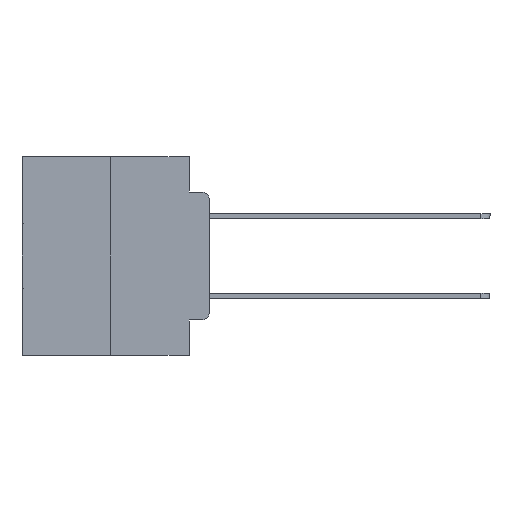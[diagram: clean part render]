
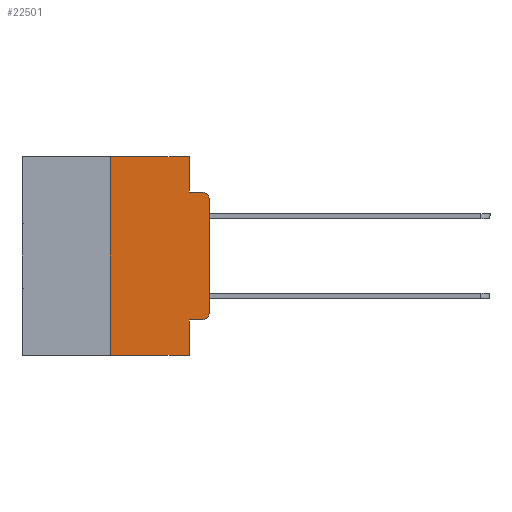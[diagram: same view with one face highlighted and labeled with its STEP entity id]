
A CAD part, left-side view. The second image highlights one B-rep face of the part: STEP entity #22501.
In plain terms, the highlighted planar face has unit normal (-1, 0, 0).
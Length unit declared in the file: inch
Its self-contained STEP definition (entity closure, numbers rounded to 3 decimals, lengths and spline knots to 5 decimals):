
#284 = CARTESIAN_POINT ( 'NONE',  ( 0., 0.051, -0.4115 ) ) ;
#371 = ORIENTED_EDGE ( 'NONE', *, *, #9940, .F. ) ;
#402 = VERTEX_POINT ( 'NONE', #22091 ) ;
#1548 = DIRECTION ( 'NONE',  ( 1., 0., 0. ) ) ;
#1615 = CIRCLE ( 'NONE', #17245, 0.02 ) ;
#2253 = EDGE_CURVE ( 'NONE', #23236, #7248, #24080, .T. ) ;
#2293 = ORIENTED_EDGE ( 'NONE', *, *, #23768, .T. ) ;
#2400 = EDGE_CURVE ( 'NONE', #23425, #27001, #1615, .T. ) ;
#2680 = ORIENTED_EDGE ( 'NONE', *, *, #15857, .F. ) ;
#2745 = DIRECTION ( 'NONE',  ( 0., -1., 0. ) ) ;
#4505 = LINE ( 'NONE', #23793, #22493 ) ;
#5071 = DIRECTION ( 'NONE',  ( 0., -1., 0. ) ) ;
#5350 = VECTOR ( 'NONE', #19750, 39.37008 ) ;
#6028 = ORIENTED_EDGE ( 'NONE', *, *, #2253, .F. ) ;
#7029 = CARTESIAN_POINT ( 'NONE',  ( 0., 0.051, 0. ) ) ;
#7248 = VERTEX_POINT ( 'NONE', #28338 ) ;
#7427 = DIRECTION ( 'NONE',  ( 0., 0., 1. ) ) ;
#7777 = VERTEX_POINT ( 'NONE', #9483 ) ;
#8182 = LINE ( 'NONE', #23609, #13715 ) ;
#9483 = CARTESIAN_POINT ( 'NONE',  ( 0., 0.051, -0.4115 ) ) ;
#9668 = DIRECTION ( 'NONE',  ( 0., 0., -1. ) ) ;
#9918 = LINE ( 'NONE', #284, #27792 ) ;
#9940 = EDGE_CURVE ( 'NONE', #402, #23236, #4505, .T. ) ;
#10490 = DIRECTION ( 'NONE',  ( -1., 0., 0. ) ) ;
#10709 = VECTOR ( 'NONE', #13813, 39.37008 ) ;
#10881 = ORIENTED_EDGE ( 'NONE', *, *, #21042, .F. ) ;
#10905 = CARTESIAN_POINT ( 'NONE',  ( 0., 0.051, -0.0885 ) ) ;
#12573 = CARTESIAN_POINT ( 'NONE',  ( 0., 0.02, -0.4115 ) ) ;
#12704 = DIRECTION ( 'NONE',  ( -1., 0., 0. ) ) ;
#13060 = VECTOR ( 'NONE', #20550, 39.37008 ) ;
#13715 = VECTOR ( 'NONE', #9668, 39.37008 ) ;
#13813 = DIRECTION ( 'NONE',  ( 0., 0., 1. ) ) ;
#13825 = LINE ( 'NONE', #7029, #25490 ) ;
#15857 = EDGE_CURVE ( 'NONE', #7777, #26980, #13825, .T. ) ;
#16709 = ORIENTED_EDGE ( 'NONE', *, *, #24658, .T. ) ;
#16712 = CARTESIAN_POINT ( 'NONE',  ( 0., 0., -0.1085 ) ) ;
#17245 = AXIS2_PLACEMENT_3D ( 'NONE', #28820, #10490, #22175 ) ;
#18044 = DIRECTION ( 'NONE',  ( 0., 0., -1. ) ) ;
#18204 = CARTESIAN_POINT ( 'NONE',  ( 0., 0.473, -0.5 ) ) ;
#18310 = EDGE_CURVE ( 'NONE', #7248, #21310, #8182, .T. ) ;
#18798 = DIRECTION ( 'NONE',  ( 0., 0., -1. ) ) ;
#19750 = DIRECTION ( 'NONE',  ( 0., -1., 0. ) ) ;
#20301 = PLANE ( 'NONE',  #23874 ) ;
#20550 = DIRECTION ( 'NONE',  ( 0., -1., 0. ) ) ;
#20642 = VERTEX_POINT ( 'NONE', #24819 ) ;
#21042 = EDGE_CURVE ( 'NONE', #21310, #20642, #28723, .T. ) ;
#21310 = VERTEX_POINT ( 'NONE', #10905 ) ;
#21402 = EDGE_CURVE ( 'NONE', #402, #26980, #25470, .T. ) ;
#22091 = CARTESIAN_POINT ( 'NONE',  ( 0., 0.25, -0.5 ) ) ;
#22175 = DIRECTION ( 'NONE',  ( 0., 0., -1. ) ) ;
#22357 = LINE ( 'NONE', #30021, #10709 ) ;
#22493 = VECTOR ( 'NONE', #7427, 39.37008 ) ;
#22501 = ADVANCED_FACE ( 'NONE', ( #27210 ), #20301, .F. ) ;
#22913 = ORIENTED_EDGE ( 'NONE', *, *, #2400, .T. ) ;
#23236 = VERTEX_POINT ( 'NONE', #25854 ) ;
#23277 = ORIENTED_EDGE ( 'NONE', *, *, #18310, .F. ) ;
#23425 = VERTEX_POINT ( 'NONE', #12573 ) ;
#23609 = CARTESIAN_POINT ( 'NONE',  ( 0., 0.051, 0. ) ) ;
#23702 = CARTESIAN_POINT ( 'NONE',  ( 0., 0., -0.3915 ) ) ;
#23768 = EDGE_CURVE ( 'NONE', #27001, #23936, #22357, .T. ) ;
#23793 = CARTESIAN_POINT ( 'NONE',  ( 0., 0.25, 0. ) ) ;
#23838 = CARTESIAN_POINT ( 'NONE',  ( 0., 0.051, -0.0885 ) ) ;
#23874 = AXIS2_PLACEMENT_3D ( 'NONE', #27361, #1548, #18044 ) ;
#23936 = VERTEX_POINT ( 'NONE', #16712 ) ;
#24080 = LINE ( 'NONE', #29841, #5350 ) ;
#24658 = EDGE_CURVE ( 'NONE', #7777, #23425, #9918, .T. ) ;
#24778 = EDGE_CURVE ( 'NONE', #23936, #20642, #25622, .T. ) ;
#24819 = CARTESIAN_POINT ( 'NONE',  ( 0., 0.02, -0.0885 ) ) ;
#25470 = LINE ( 'NONE', #18204, #13060 ) ;
#25490 = VECTOR ( 'NONE', #18798, 39.37008 ) ;
#25622 = CIRCLE ( 'NONE', #26080, 0.02 ) ;
#25854 = CARTESIAN_POINT ( 'NONE',  ( 0., 0.25, 0. ) ) ;
#26080 = AXIS2_PLACEMENT_3D ( 'NONE', #26683, #12704, #28994 ) ;
#26465 = EDGE_LOOP ( 'NONE', ( #2293, #28025, #10881, #23277, #6028, #371, #26940, #2680, #16709, #22913 ) ) ;
#26683 = CARTESIAN_POINT ( 'NONE',  ( 0., 0.02, -0.1085 ) ) ;
#26940 = ORIENTED_EDGE ( 'NONE', *, *, #21402, .T. ) ;
#26980 = VERTEX_POINT ( 'NONE', #28296 ) ;
#27001 = VERTEX_POINT ( 'NONE', #23702 ) ;
#27210 = FACE_OUTER_BOUND ( 'NONE', #26465, .T. ) ;
#27361 = CARTESIAN_POINT ( 'NONE',  ( 0., 0.473, 0. ) ) ;
#27792 = VECTOR ( 'NONE', #2745, 39.37008 ) ;
#28024 = VECTOR ( 'NONE', #5071, 39.37008 ) ;
#28025 = ORIENTED_EDGE ( 'NONE', *, *, #24778, .T. ) ;
#28296 = CARTESIAN_POINT ( 'NONE',  ( 0., 0.051, -0.5 ) ) ;
#28338 = CARTESIAN_POINT ( 'NONE',  ( 0., 0.051, 0. ) ) ;
#28723 = LINE ( 'NONE', #23838, #28024 ) ;
#28820 = CARTESIAN_POINT ( 'NONE',  ( 0., 0.02, -0.3915 ) ) ;
#28994 = DIRECTION ( 'NONE',  ( 0., 0., -1. ) ) ;
#29841 = CARTESIAN_POINT ( 'NONE',  ( 0., 0.473, 0. ) ) ;
#30021 = CARTESIAN_POINT ( 'NONE',  ( 0., 0., 0. ) ) ;
